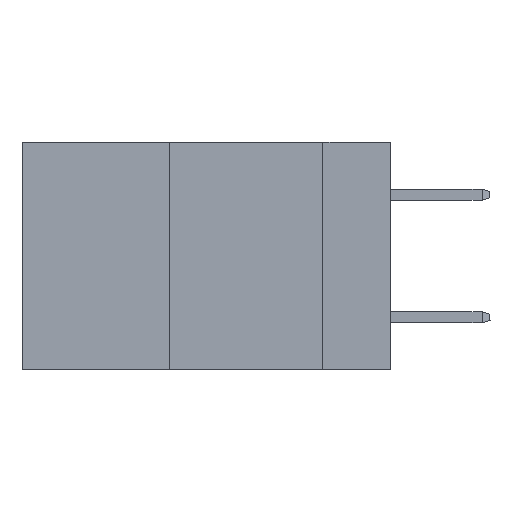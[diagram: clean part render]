
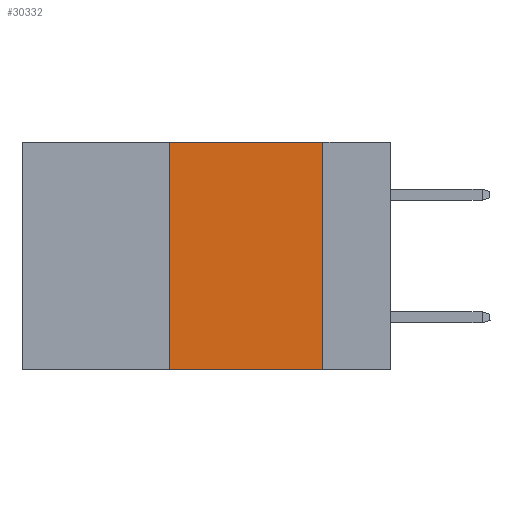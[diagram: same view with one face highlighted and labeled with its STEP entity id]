
A CAD part, left-side view. The second image highlights one B-rep face of the part: STEP entity #30332.
In plain terms, the highlighted planar face has unit normal (-1, 0, 0).
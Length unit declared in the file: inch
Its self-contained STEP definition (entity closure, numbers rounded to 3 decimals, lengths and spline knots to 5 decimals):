
#407 = CARTESIAN_POINT ( 'NONE',  ( 0., 0.11, 0. ) ) ;
#953 = CARTESIAN_POINT ( 'NONE',  ( 0., 0.6, -0.37 ) ) ;
#1533 = VECTOR ( 'NONE', #36371, 39.37008 ) ;
#1717 = LINE ( 'NONE', #33829, #24919 ) ;
#2196 = EDGE_CURVE ( 'NONE', #4974, #17461, #8511, .T. ) ;
#4974 = VERTEX_POINT ( 'NONE', #33148 ) ;
#5540 = CARTESIAN_POINT ( 'NONE',  ( 0., 0.36, 0. ) ) ;
#6523 = ORIENTED_EDGE ( 'NONE', *, *, #27724, .F. ) ;
#6920 = ORIENTED_EDGE ( 'NONE', *, *, #2196, .F. ) ;
#8511 = LINE ( 'NONE', #39684, #31646 ) ;
#8655 = FACE_OUTER_BOUND ( 'NONE', #20190, .T. ) ;
#10220 = DIRECTION ( 'NONE',  ( 0., 0., -1. ) ) ;
#13583 = VERTEX_POINT ( 'NONE', #40305 ) ;
#17399 = CARTESIAN_POINT ( 'NONE',  ( 0., 0.6, 0. ) ) ;
#17461 = VERTEX_POINT ( 'NONE', #5540 ) ;
#18827 = EDGE_CURVE ( 'NONE', #4974, #13583, #27491, .T. ) ;
#20190 = EDGE_LOOP ( 'NONE', ( #6523, #21441, #6920, #22113 ) ) ;
#21441 = ORIENTED_EDGE ( 'NONE', *, *, #31935, .F. ) ;
#22113 = ORIENTED_EDGE ( 'NONE', *, *, #18827, .T. ) ;
#23194 = LINE ( 'NONE', #17399, #1533 ) ;
#23874 = DIRECTION ( 'NONE',  ( 0., 0., 1. ) ) ;
#24919 = VECTOR ( 'NONE', #10220, 39.37008 ) ;
#25019 = DIRECTION ( 'NONE',  ( 0., 0., -1. ) ) ;
#25294 = DIRECTION ( 'NONE',  ( 1., 0., 0. ) ) ;
#27491 = LINE ( 'NONE', #953, #41556 ) ;
#27724 = EDGE_CURVE ( 'NONE', #29990, #13583, #1717, .T. ) ;
#27947 = CARTESIAN_POINT ( 'NONE',  ( 0., 0.6, 0. ) ) ;
#29990 = VERTEX_POINT ( 'NONE', #407 ) ;
#30332 = ADVANCED_FACE ( 'NONE', ( #8655 ), #34409, .F. ) ;
#30620 = AXIS2_PLACEMENT_3D ( 'NONE', #27947, #25294, #25019 ) ;
#31646 = VECTOR ( 'NONE', #23874, 39.37008 ) ;
#31935 = EDGE_CURVE ( 'NONE', #17461, #29990, #23194, .T. ) ;
#33148 = CARTESIAN_POINT ( 'NONE',  ( 0., 0.36, -0.37 ) ) ;
#33829 = CARTESIAN_POINT ( 'NONE',  ( 0., 0.11, 0. ) ) ;
#34409 = PLANE ( 'NONE',  #30620 ) ;
#36371 = DIRECTION ( 'NONE',  ( 0., -1., 0. ) ) ;
#39588 = DIRECTION ( 'NONE',  ( 0., -1., 0. ) ) ;
#39684 = CARTESIAN_POINT ( 'NONE',  ( 0., 0.36, 0. ) ) ;
#40305 = CARTESIAN_POINT ( 'NONE',  ( 0., 0.11, -0.37 ) ) ;
#41556 = VECTOR ( 'NONE', #39588, 39.37008 ) ;
